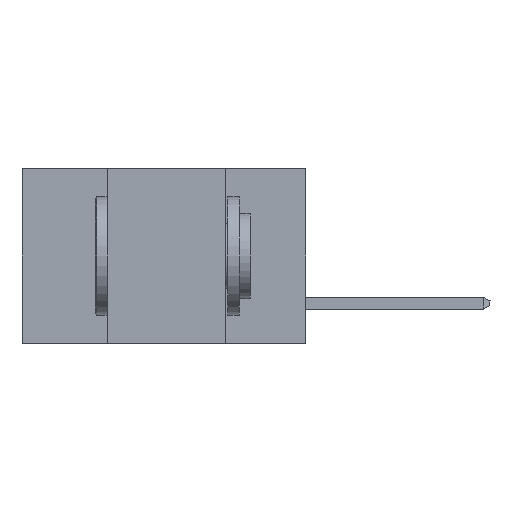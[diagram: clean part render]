
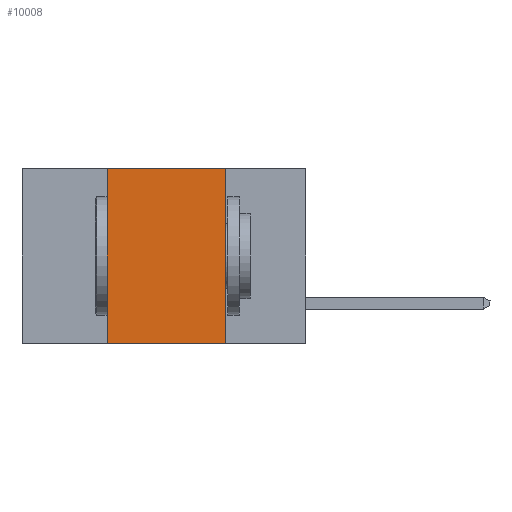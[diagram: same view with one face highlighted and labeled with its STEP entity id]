
A CAD part, left-side view. The second image highlights one B-rep face of the part: STEP entity #10008.
In plain terms, the highlighted planar face has unit normal (-1, 0, 0).
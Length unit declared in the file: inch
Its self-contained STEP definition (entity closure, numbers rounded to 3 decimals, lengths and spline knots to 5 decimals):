
#494 = CARTESIAN_POINT ( 'NONE',  ( 0., 0.6, -0.37 ) ) ;
#1295 = VERTEX_POINT ( 'NONE', #10721 ) ;
#1321 = CARTESIAN_POINT ( 'NONE',  ( 0., 0.42, -0.37 ) ) ;
#1509 = DIRECTION ( 'NONE',  ( 1., 0., 0. ) ) ;
#1647 = LINE ( 'NONE', #494, #9841 ) ;
#2009 = LINE ( 'NONE', #6156, #2081 ) ;
#2081 = VECTOR ( 'NONE', #9620, 39.37008 ) ;
#2858 = EDGE_CURVE ( 'NONE', #4439, #9736, #1647, .T. ) ;
#3735 = ORIENTED_EDGE ( 'NONE', *, *, #5725, .F. ) ;
#4439 = VERTEX_POINT ( 'NONE', #11023 ) ;
#4832 = EDGE_CURVE ( 'NONE', #4439, #1295, #12392, .T. ) ;
#5725 = EDGE_CURVE ( 'NONE', #1295, #10574, #13864, .T. ) ;
#5841 = DIRECTION ( 'NONE',  ( 0., 0., -1. ) ) ;
#6112 = DIRECTION ( 'NONE',  ( 0., -1., 0. ) ) ;
#6156 = CARTESIAN_POINT ( 'NONE',  ( 0., 0.17, -0.37 ) ) ;
#6189 = VECTOR ( 'NONE', #10366, 39.37008 ) ;
#6571 = AXIS2_PLACEMENT_3D ( 'NONE', #11476, #1509, #5841 ) ;
#7442 = EDGE_CURVE ( 'NONE', #10574, #9736, #2009, .T. ) ;
#8543 = CARTESIAN_POINT ( 'NONE',  ( 0., 0.17, -0.37 ) ) ;
#9333 = CARTESIAN_POINT ( 'NONE',  ( 0., 0.6, 0. ) ) ;
#9620 = DIRECTION ( 'NONE',  ( 0., 0., -1. ) ) ;
#9736 = VERTEX_POINT ( 'NONE', #8543 ) ;
#9841 = VECTOR ( 'NONE', #6112, 39.37008 ) ;
#9913 = ORIENTED_EDGE ( 'NONE', *, *, #2858, .T. ) ;
#10008 = ADVANCED_FACE ( 'NONE', ( #13763 ), #10122, .F. ) ;
#10122 = PLANE ( 'NONE',  #6571 ) ;
#10202 = ORIENTED_EDGE ( 'NONE', *, *, #7442, .F. ) ;
#10293 = DIRECTION ( 'NONE',  ( 0., -1., 0. ) ) ;
#10325 = CARTESIAN_POINT ( 'NONE',  ( 0., 0.17, 0. ) ) ;
#10366 = DIRECTION ( 'NONE',  ( 0., 0., 1. ) ) ;
#10574 = VERTEX_POINT ( 'NONE', #10325 ) ;
#10721 = CARTESIAN_POINT ( 'NONE',  ( 0., 0.42, 0. ) ) ;
#10942 = EDGE_LOOP ( 'NONE', ( #10202, #3735, #13060, #9913 ) ) ;
#11023 = CARTESIAN_POINT ( 'NONE',  ( 0., 0.42, -0.37 ) ) ;
#11476 = CARTESIAN_POINT ( 'NONE',  ( 0., 0.6, 0. ) ) ;
#12392 = LINE ( 'NONE', #1321, #6189 ) ;
#13060 = ORIENTED_EDGE ( 'NONE', *, *, #4832, .F. ) ;
#13763 = FACE_OUTER_BOUND ( 'NONE', #10942, .T. ) ;
#13864 = LINE ( 'NONE', #9333, #14109 ) ;
#14109 = VECTOR ( 'NONE', #10293, 39.37008 ) ;
